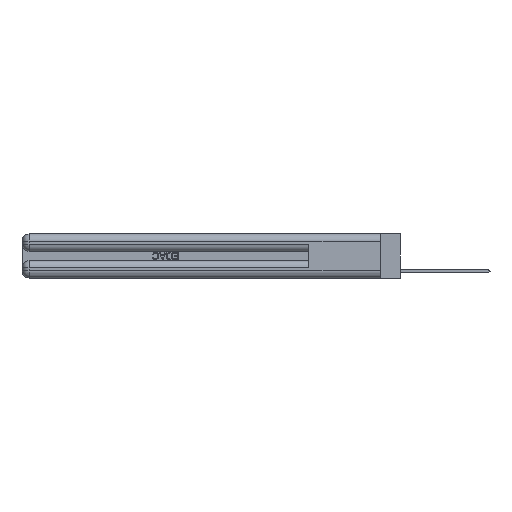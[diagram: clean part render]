
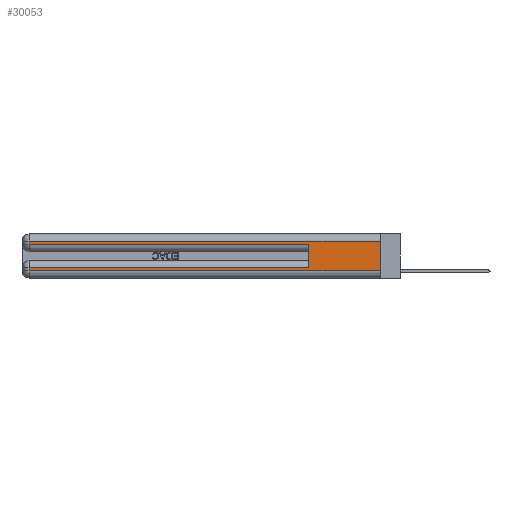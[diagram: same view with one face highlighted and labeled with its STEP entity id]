
A CAD part, left-side view. The second image highlights one B-rep face of the part: STEP entity #30053.
In plain terms, the highlighted planar face has unit normal (-1, 0, 0).
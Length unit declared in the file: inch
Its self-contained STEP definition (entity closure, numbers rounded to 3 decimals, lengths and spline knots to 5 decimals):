
#297 = VECTOR ( 'NONE', #17912, 39.37008 ) ;
#481 = CARTESIAN_POINT ( 'NONE',  ( 0., 0., 0.285 ) ) ;
#702 = VECTOR ( 'NONE', #28165, 39.37008 ) ;
#861 = VERTEX_POINT ( 'NONE', #20450 ) ;
#1219 = CARTESIAN_POINT ( 'NONE',  ( 0., 0., 0.06 ) ) ;
#1282 = EDGE_LOOP ( 'NONE', ( #5461, #31881, #6055, #17615, #30436, #23701, #4775, #30337 ) ) ;
#1722 = DIRECTION ( 'NONE',  ( 0., 1., 0. ) ) ;
#1966 = CARTESIAN_POINT ( 'NONE',  ( 0., 2.94, 0.085 ) ) ;
#1992 = CARTESIAN_POINT ( 'NONE',  ( 0., 0.6, 0.085 ) ) ;
#2300 = LINE ( 'NONE', #20949, #3128 ) ;
#3128 = VECTOR ( 'NONE', #20282, 39.37008 ) ;
#4775 = ORIENTED_EDGE ( 'NONE', *, *, #31330, .T. ) ;
#5461 = ORIENTED_EDGE ( 'NONE', *, *, #7342, .F. ) ;
#6055 = ORIENTED_EDGE ( 'NONE', *, *, #18531, .T. ) ;
#6266 = CARTESIAN_POINT ( 'NONE',  ( 0., 2.94, 0.285 ) ) ;
#7342 = EDGE_CURVE ( 'NONE', #33427, #21602, #2300, .T. ) ;
#7755 = VECTOR ( 'NONE', #19180, 39.37008 ) ;
#8287 = AXIS2_PLACEMENT_3D ( 'NONE', #33807, #17400, #17753 ) ;
#11367 = CARTESIAN_POINT ( 'NONE',  ( 0., 0.6, 0.145 ) ) ;
#11581 = CARTESIAN_POINT ( 'NONE',  ( 0., 0.6, 0.285 ) ) ;
#12451 = LINE ( 'NONE', #33434, #702 ) ;
#12733 = EDGE_CURVE ( 'NONE', #861, #21602, #32626, .T. ) ;
#12852 = EDGE_CURVE ( 'NONE', #33427, #14814, #12451, .T. ) ;
#13348 = DIRECTION ( 'NONE',  ( 0., 0., -1. ) ) ;
#14585 = PLANE ( 'NONE',  #8287 ) ;
#14814 = VERTEX_POINT ( 'NONE', #19824 ) ;
#15031 = LINE ( 'NONE', #33676, #29341 ) ;
#15759 = CARTESIAN_POINT ( 'NONE',  ( 0., 0., 0.31 ) ) ;
#16391 = VERTEX_POINT ( 'NONE', #1992 ) ;
#16781 = DIRECTION ( 'NONE',  ( 0., 0., 1. ) ) ;
#17367 = VECTOR ( 'NONE', #29084, 39.37008 ) ;
#17400 = DIRECTION ( 'NONE',  ( 1., 0., 0. ) ) ;
#17615 = ORIENTED_EDGE ( 'NONE', *, *, #29945, .T. ) ;
#17753 = DIRECTION ( 'NONE',  ( 0., 0., -1. ) ) ;
#17912 = DIRECTION ( 'NONE',  ( 0., -1., 0. ) ) ;
#18531 = EDGE_CURVE ( 'NONE', #14814, #31135, #24675, .T. ) ;
#19057 = LINE ( 'NONE', #26446, #17367 ) ;
#19180 = DIRECTION ( 'NONE',  ( 0., -1., 0. ) ) ;
#19824 = CARTESIAN_POINT ( 'NONE',  ( 0., 2.94, 0.31 ) ) ;
#20282 = DIRECTION ( 'NONE',  ( 0., 0., -1. ) ) ;
#20300 = EDGE_CURVE ( 'NONE', #16391, #25828, #15031, .T. ) ;
#20450 = CARTESIAN_POINT ( 'NONE',  ( 0., 2.94, 0.06 ) ) ;
#20949 = CARTESIAN_POINT ( 'NONE',  ( 0., 0., 0.37 ) ) ;
#21340 = VECTOR ( 'NONE', #13348, 39.37008 ) ;
#21602 = VERTEX_POINT ( 'NONE', #22295 ) ;
#22295 = CARTESIAN_POINT ( 'NONE',  ( 0., 0., 0.06 ) ) ;
#22332 = VECTOR ( 'NONE', #16781, 39.37008 ) ;
#23701 = ORIENTED_EDGE ( 'NONE', *, *, #20300, .T. ) ;
#24130 = LINE ( 'NONE', #481, #7755 ) ;
#24675 = LINE ( 'NONE', #29467, #21340 ) ;
#25807 = FACE_OUTER_BOUND ( 'NONE', #1282, .T. ) ;
#25828 = VERTEX_POINT ( 'NONE', #1966 ) ;
#26446 = CARTESIAN_POINT ( 'NONE',  ( 0., 2.94, 0.37 ) ) ;
#28165 = DIRECTION ( 'NONE',  ( 0., 1., 0. ) ) ;
#28615 = LINE ( 'NONE', #11367, #22332 ) ;
#29084 = DIRECTION ( 'NONE',  ( 0., 0., -1. ) ) ;
#29341 = VECTOR ( 'NONE', #1722, 39.37008 ) ;
#29467 = CARTESIAN_POINT ( 'NONE',  ( 0., 2.94, 0.37 ) ) ;
#29865 = VERTEX_POINT ( 'NONE', #11581 ) ;
#29945 = EDGE_CURVE ( 'NONE', #31135, #29865, #24130, .T. ) ;
#30053 = ADVANCED_FACE ( 'NONE', ( #25807 ), #14585, .F. ) ;
#30337 = ORIENTED_EDGE ( 'NONE', *, *, #12733, .T. ) ;
#30436 = ORIENTED_EDGE ( 'NONE', *, *, #32439, .F. ) ;
#31135 = VERTEX_POINT ( 'NONE', #6266 ) ;
#31330 = EDGE_CURVE ( 'NONE', #25828, #861, #19057, .T. ) ;
#31881 = ORIENTED_EDGE ( 'NONE', *, *, #12852, .T. ) ;
#32439 = EDGE_CURVE ( 'NONE', #16391, #29865, #28615, .T. ) ;
#32626 = LINE ( 'NONE', #1219, #297 ) ;
#33427 = VERTEX_POINT ( 'NONE', #15759 ) ;
#33434 = CARTESIAN_POINT ( 'NONE',  ( 0., 0., 0.31 ) ) ;
#33676 = CARTESIAN_POINT ( 'NONE',  ( 0., 0., 0.085 ) ) ;
#33807 = CARTESIAN_POINT ( 'NONE',  ( 0., 0., 0.37 ) ) ;
